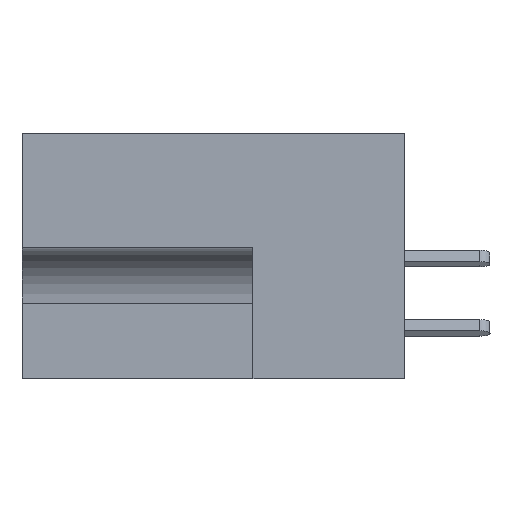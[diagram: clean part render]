
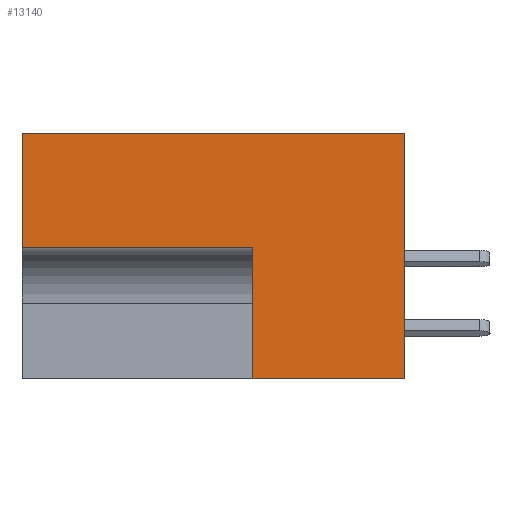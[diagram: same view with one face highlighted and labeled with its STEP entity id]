
A CAD part, left-side view. The second image highlights one B-rep face of the part: STEP entity #13140.
In plain terms, the highlighted planar face has unit normal (-1, 0, 0).
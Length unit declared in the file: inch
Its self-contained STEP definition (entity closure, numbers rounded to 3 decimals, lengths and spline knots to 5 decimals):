
#1311 = CARTESIAN_POINT ( 'NONE',  ( 0., 0.328, -0.248 ) ) ;
#1896 = PLANE ( 'NONE',  #12795 ) ;
#1965 = DIRECTION ( 'NONE',  ( 1., 0., 0. ) ) ;
#2116 = CARTESIAN_POINT ( 'NONE',  ( 0., 0.328, -0.248 ) ) ;
#2780 = LINE ( 'NONE', #11648, #10447 ) ;
#3385 = LINE ( 'NONE', #4401, #13279 ) ;
#3477 = DIRECTION ( 'NONE',  ( 0., -1., 0. ) ) ;
#3651 = VECTOR ( 'NONE', #12096, 39.37008 ) ;
#4401 = CARTESIAN_POINT ( 'NONE',  ( 0., 0.453, -0.531 ) ) ;
#4927 = LINE ( 'NONE', #2116, #3651 ) ;
#5103 = EDGE_CURVE ( 'NONE', #16623, #9111, #6685, .T. ) ;
#5383 = LINE ( 'NONE', #16518, #18328 ) ;
#6215 = EDGE_LOOP ( 'NONE', ( #19316, #11329, #13962, #9644, #17218, #9832 ) ) ;
#6685 = LINE ( 'NONE', #9371, #8210 ) ;
#7447 = EDGE_CURVE ( 'NONE', #11930, #8605, #2780, .T. ) ;
#7680 = CARTESIAN_POINT ( 'NONE',  ( 0., 0.828, 0. ) ) ;
#8210 = VECTOR ( 'NONE', #19131, 39.37008 ) ;
#8375 = DIRECTION ( 'NONE',  ( 0., 0., 1. ) ) ;
#8605 = VERTEX_POINT ( 'NONE', #7680 ) ;
#9111 = VERTEX_POINT ( 'NONE', #13816 ) ;
#9371 = CARTESIAN_POINT ( 'NONE',  ( 0., 0., 0. ) ) ;
#9644 = ORIENTED_EDGE ( 'NONE', *, *, #20982, .T. ) ;
#9832 = ORIENTED_EDGE ( 'NONE', *, *, #14260, .F. ) ;
#10447 = VECTOR ( 'NONE', #14756, 39.37008 ) ;
#11329 = ORIENTED_EDGE ( 'NONE', *, *, #13179, .F. ) ;
#11415 = VERTEX_POINT ( 'NONE', #1311 ) ;
#11648 = CARTESIAN_POINT ( 'NONE',  ( 0., 0.828, 0. ) ) ;
#11930 = VERTEX_POINT ( 'NONE', #15459 ) ;
#12096 = DIRECTION ( 'NONE',  ( 0., 1., 0. ) ) ;
#12795 = AXIS2_PLACEMENT_3D ( 'NONE', #18246, #1965, #16676 ) ;
#13140 = ADVANCED_FACE ( 'NONE', ( #19628 ), #1896, .F. ) ;
#13179 = EDGE_CURVE ( 'NONE', #11415, #11930, #4927, .T. ) ;
#13279 = VECTOR ( 'NONE', #18942, 39.37008 ) ;
#13537 = EDGE_CURVE ( 'NONE', #16710, #11415, #19847, .T. ) ;
#13816 = CARTESIAN_POINT ( 'NONE',  ( 0., 0., 0. ) ) ;
#13962 = ORIENTED_EDGE ( 'NONE', *, *, #13537, .F. ) ;
#14260 = EDGE_CURVE ( 'NONE', #8605, #9111, #5383, .T. ) ;
#14349 = CARTESIAN_POINT ( 'NONE',  ( 0., 0., -0.531 ) ) ;
#14627 = CARTESIAN_POINT ( 'NONE',  ( 0., 0.328, -0.531 ) ) ;
#14756 = DIRECTION ( 'NONE',  ( 0., 0., 1. ) ) ;
#15459 = CARTESIAN_POINT ( 'NONE',  ( 0., 0.828, -0.248 ) ) ;
#16518 = CARTESIAN_POINT ( 'NONE',  ( 0., 0.453, 0. ) ) ;
#16623 = VERTEX_POINT ( 'NONE', #14349 ) ;
#16676 = DIRECTION ( 'NONE',  ( 0., 0., -1. ) ) ;
#16710 = VERTEX_POINT ( 'NONE', #14627 ) ;
#17218 = ORIENTED_EDGE ( 'NONE', *, *, #5103, .T. ) ;
#17948 = CARTESIAN_POINT ( 'NONE',  ( 0., 0.328, -0.531 ) ) ;
#18246 = CARTESIAN_POINT ( 'NONE',  ( 0., 0.453, 0. ) ) ;
#18328 = VECTOR ( 'NONE', #3477, 39.37008 ) ;
#18942 = DIRECTION ( 'NONE',  ( 0., -1., 0. ) ) ;
#19131 = DIRECTION ( 'NONE',  ( 0., 0., 1. ) ) ;
#19316 = ORIENTED_EDGE ( 'NONE', *, *, #7447, .F. ) ;
#19628 = FACE_OUTER_BOUND ( 'NONE', #6215, .T. ) ;
#19847 = LINE ( 'NONE', #17948, #20871 ) ;
#20871 = VECTOR ( 'NONE', #8375, 39.37008 ) ;
#20982 = EDGE_CURVE ( 'NONE', #16710, #16623, #3385, .T. ) ;
